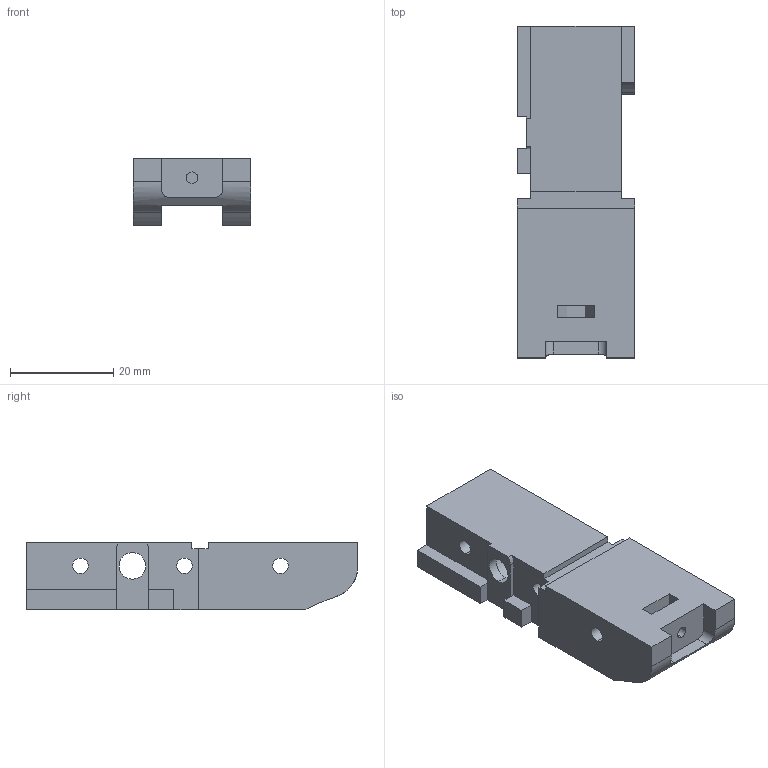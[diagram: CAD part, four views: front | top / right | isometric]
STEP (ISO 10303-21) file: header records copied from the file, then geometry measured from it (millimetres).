
FILE_DESCRIPTION (( 'STEP AP214' ), '1' );
FILE_NAME ('Reinforced_Mag_Well_Rear.step', '2015-06-12T17:09:04', ( '' ), ( '' ), 'SwSTEP 2.0', 'SolidWorks 2015', '' );
FILE_SCHEMA (( 'AUTOMOTIVE_DESIGN' ));
Length unit declared in the file: millimetre
Products named in the file (1): Reinforced_Mag_Well_Rear
Bounding box: 22.81 x 64.36 x 13.13 mm (x, y, z)
Volume: 11860.8 mm3; surface area: 6611.6 mm2
Topology: 1 solids, 1 shells, 71 faces, 195 edges, 128 vertices
Faces by surface type: plane 48, cylinder 23
Entity records: 2325 total; most frequent: CARTESIAN_POINT 421, ORIENTED_EDGE 390, DIRECTION 385, EDGE_CURVE 195, LINE 145, VECTOR 145, VERTEX_POINT 128, AXIS2_PLACEMENT_3D 120
